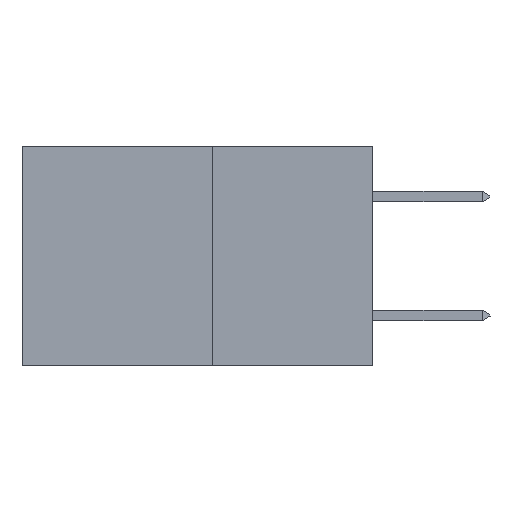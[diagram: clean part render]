
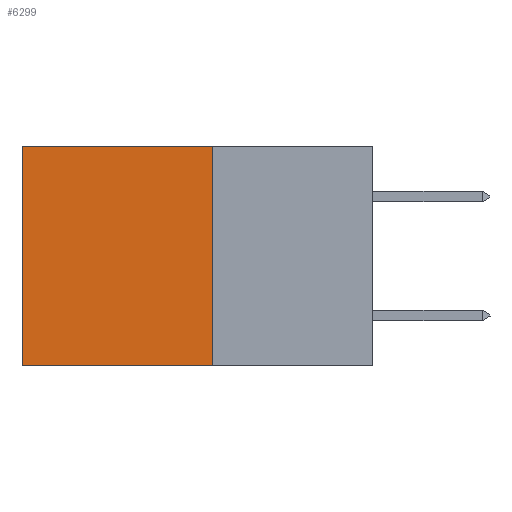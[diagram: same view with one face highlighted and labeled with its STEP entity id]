
A CAD part, left-side view. The second image highlights one B-rep face of the part: STEP entity #6299.
In plain terms, the highlighted planar face has unit normal (-1, 0, 0).
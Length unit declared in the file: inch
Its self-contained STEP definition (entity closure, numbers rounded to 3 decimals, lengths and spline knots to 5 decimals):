
#499 = VECTOR ( 'NONE', #3744, 39.37008 ) ;
#560 = VECTOR ( 'NONE', #11134, 39.37008 ) ;
#851 = CARTESIAN_POINT ( 'NONE',  ( 0.277, 0.27, -0.37 ) ) ;
#1413 = EDGE_CURVE ( 'NONE', #7681, #11339, #2828, .T. ) ;
#1954 = DIRECTION ( 'NONE',  ( 0., 1., 0. ) ) ;
#2125 = PLANE ( 'NONE',  #10747 ) ;
#2446 = EDGE_CURVE ( 'NONE', #9443, #7681, #3239, .T. ) ;
#2504 = CARTESIAN_POINT ( 'NONE',  ( 0.277, 0.27, -0.37 ) ) ;
#2578 = DIRECTION ( 'NONE',  ( 0., 0., -1. ) ) ;
#2655 = CARTESIAN_POINT ( 'NONE',  ( 0.277, 0.27, 0. ) ) ;
#2828 = LINE ( 'NONE', #2504, #6890 ) ;
#3096 = CARTESIAN_POINT ( 'NONE',  ( 0.277, 0.27, -0.37 ) ) ;
#3183 = LINE ( 'NONE', #9808, #499 ) ;
#3239 = LINE ( 'NONE', #11158, #560 ) ;
#3744 = DIRECTION ( 'NONE',  ( 0., 1., 0. ) ) ;
#4072 = DIRECTION ( 'NONE',  ( 0., 0., -1. ) ) ;
#4463 = EDGE_CURVE ( 'NONE', #9443, #9392, #3183, .T. ) ;
#5227 = EDGE_CURVE ( 'NONE', #9392, #11339, #5567, .T. ) ;
#5464 = CARTESIAN_POINT ( 'NONE',  ( 0.277, 0.59, -0.37 ) ) ;
#5567 = LINE ( 'NONE', #5464, #7880 ) ;
#6299 = ADVANCED_FACE ( 'NONE', ( #10612 ), #2125, .F. ) ;
#6890 = VECTOR ( 'NONE', #1954, 39.37008 ) ;
#7681 = VERTEX_POINT ( 'NONE', #851 ) ;
#7758 = ORIENTED_EDGE ( 'NONE', *, *, #2446, .F. ) ;
#7880 = VECTOR ( 'NONE', #2578, 39.37008 ) ;
#7907 = CARTESIAN_POINT ( 'NONE',  ( 0.277, 0.59, -0.37 ) ) ;
#8912 = CARTESIAN_POINT ( 'NONE',  ( 0.277, 0.59, 0. ) ) ;
#9336 = DIRECTION ( 'NONE',  ( 1., 0., 0. ) ) ;
#9342 = EDGE_LOOP ( 'NONE', ( #11493, #9682, #7758, #9925 ) ) ;
#9392 = VERTEX_POINT ( 'NONE', #8912 ) ;
#9443 = VERTEX_POINT ( 'NONE', #2655 ) ;
#9682 = ORIENTED_EDGE ( 'NONE', *, *, #1413, .F. ) ;
#9808 = CARTESIAN_POINT ( 'NONE',  ( 0.277, 0.27, 0. ) ) ;
#9925 = ORIENTED_EDGE ( 'NONE', *, *, #4463, .T. ) ;
#10612 = FACE_OUTER_BOUND ( 'NONE', #9342, .T. ) ;
#10747 = AXIS2_PLACEMENT_3D ( 'NONE', #3096, #9336, #4072 ) ;
#11134 = DIRECTION ( 'NONE',  ( 0., 0., -1. ) ) ;
#11158 = CARTESIAN_POINT ( 'NONE',  ( 0.277, 0.27, -0.37 ) ) ;
#11339 = VERTEX_POINT ( 'NONE', #7907 ) ;
#11493 = ORIENTED_EDGE ( 'NONE', *, *, #5227, .T. ) ;
